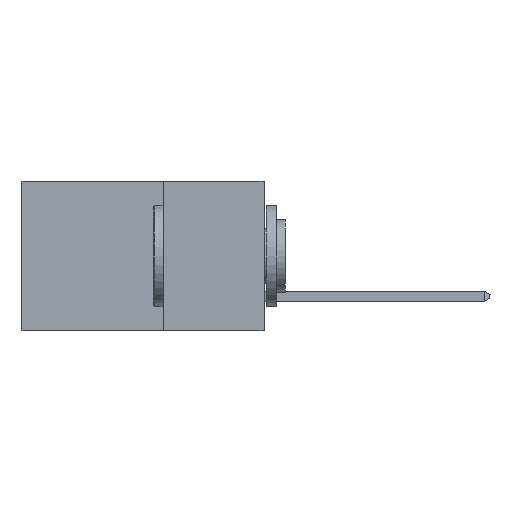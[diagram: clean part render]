
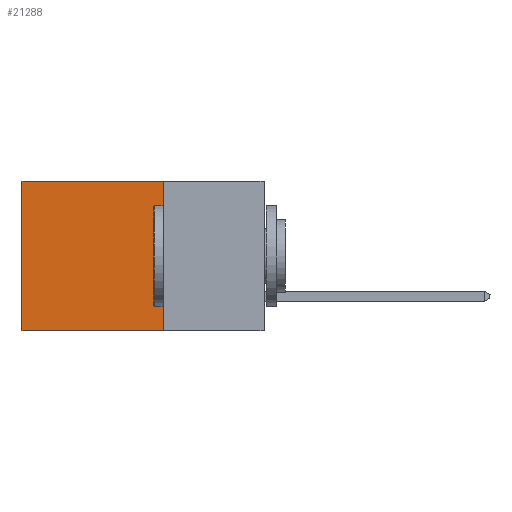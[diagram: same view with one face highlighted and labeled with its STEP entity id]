
A CAD part, left-side view. The second image highlights one B-rep face of the part: STEP entity #21288.
In plain terms, the highlighted planar face has unit normal (-1, 0, 0).
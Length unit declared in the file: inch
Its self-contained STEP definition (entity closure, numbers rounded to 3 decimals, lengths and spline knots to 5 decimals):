
#2346 = CARTESIAN_POINT ( 'NONE',  ( 0.2615, 0.25, -0.37 ) ) ;
#2438 = EDGE_CURVE ( 'NONE', #11796, #24879, #15987, .T. ) ;
#2467 = EDGE_LOOP ( 'NONE', ( #25619, #7876, #10972, #12905 ) ) ;
#2491 = DIRECTION ( 'NONE',  ( 1., 0., 0. ) ) ;
#2758 = DIRECTION ( 'NONE',  ( 0., 0., -1. ) ) ;
#3017 = CARTESIAN_POINT ( 'NONE',  ( 0.2615, 0.25, -0.37 ) ) ;
#3114 = VECTOR ( 'NONE', #18066, 39.37008 ) ;
#4197 = CARTESIAN_POINT ( 'NONE',  ( 0.2615, 0.6, -0.37 ) ) ;
#4360 = LINE ( 'NONE', #2346, #15161 ) ;
#4491 = CARTESIAN_POINT ( 'NONE',  ( 0.2615, 0.6, 0. ) ) ;
#7876 = ORIENTED_EDGE ( 'NONE', *, *, #11026, .F. ) ;
#9570 = CARTESIAN_POINT ( 'NONE',  ( 0.2615, 0.25, 0. ) ) ;
#10972 = ORIENTED_EDGE ( 'NONE', *, *, #14830, .F. ) ;
#11026 = EDGE_CURVE ( 'NONE', #22969, #25775, #4360, .T. ) ;
#11796 = VERTEX_POINT ( 'NONE', #9570 ) ;
#11984 = DIRECTION ( 'NONE',  ( 0., 1., 0. ) ) ;
#12331 = LINE ( 'NONE', #18856, #24181 ) ;
#12905 = ORIENTED_EDGE ( 'NONE', *, *, #2438, .T. ) ;
#13058 = CARTESIAN_POINT ( 'NONE',  ( 0.2615, 0.6, -0.37 ) ) ;
#13915 = VECTOR ( 'NONE', #11984, 39.37008 ) ;
#14830 = EDGE_CURVE ( 'NONE', #11796, #22969, #12331, .T. ) ;
#15150 = DIRECTION ( 'NONE',  ( 0., 1., 0. ) ) ;
#15161 = VECTOR ( 'NONE', #15150, 39.37008 ) ;
#15770 = AXIS2_PLACEMENT_3D ( 'NONE', #3017, #2491, #2758 ) ;
#15987 = LINE ( 'NONE', #25853, #13915 ) ;
#18066 = DIRECTION ( 'NONE',  ( 0., 0., -1. ) ) ;
#18466 = DIRECTION ( 'NONE',  ( 0., 0., -1. ) ) ;
#18772 = FACE_OUTER_BOUND ( 'NONE', #2467, .T. ) ;
#18856 = CARTESIAN_POINT ( 'NONE',  ( 0.2615, 0.25, -0.37 ) ) ;
#21038 = PLANE ( 'NONE',  #15770 ) ;
#21288 = ADVANCED_FACE ( 'NONE', ( #18772 ), #21038, .F. ) ;
#22457 = LINE ( 'NONE', #4197, #3114 ) ;
#22969 = VERTEX_POINT ( 'NONE', #25133 ) ;
#24181 = VECTOR ( 'NONE', #18466, 39.37008 ) ;
#24879 = VERTEX_POINT ( 'NONE', #4491 ) ;
#25133 = CARTESIAN_POINT ( 'NONE',  ( 0.2615, 0.25, -0.37 ) ) ;
#25190 = EDGE_CURVE ( 'NONE', #24879, #25775, #22457, .T. ) ;
#25619 = ORIENTED_EDGE ( 'NONE', *, *, #25190, .T. ) ;
#25775 = VERTEX_POINT ( 'NONE', #13058 ) ;
#25853 = CARTESIAN_POINT ( 'NONE',  ( 0.2615, 0.25, 0. ) ) ;
